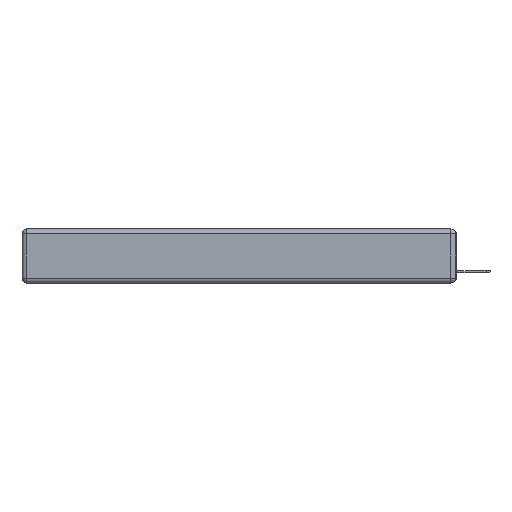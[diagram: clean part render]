
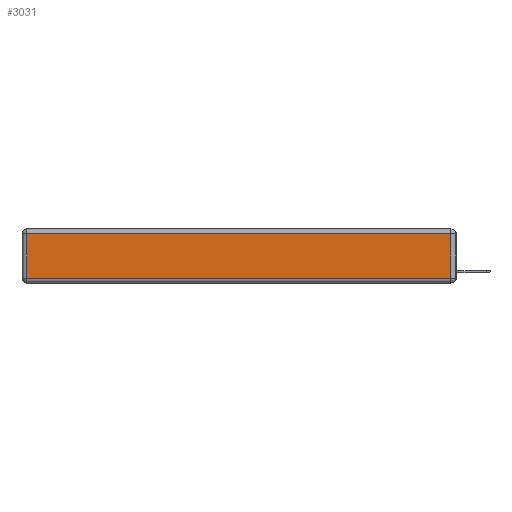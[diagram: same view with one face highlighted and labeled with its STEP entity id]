
A CAD part, left-side view. The second image highlights one B-rep face of the part: STEP entity #3031.
In plain terms, the highlighted planar face has unit normal (-1, 0, 0).
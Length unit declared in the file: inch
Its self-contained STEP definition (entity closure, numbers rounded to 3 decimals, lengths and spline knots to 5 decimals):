
#930 = CARTESIAN_POINT ( 'NONE',  ( 0., 2.72, -0.343 ) ) ;
#2395 = LINE ( 'NONE', #15706, #4545 ) ;
#2981 = ORIENTED_EDGE ( 'NONE', *, *, #5300, .T. ) ;
#3031 = ADVANCED_FACE ( 'NONE', ( #9175 ), #5121, .T. ) ;
#3174 = CARTESIAN_POINT ( 'NONE',  ( 0., 2.75, -0.03 ) ) ;
#3621 = DIRECTION ( 'NONE',  ( 0., 0., 1. ) ) ;
#4376 = VECTOR ( 'NONE', #15679, 39.37008 ) ;
#4486 = VERTEX_POINT ( 'NONE', #12995 ) ;
#4545 = VECTOR ( 'NONE', #3621, 39.37008 ) ;
#4649 = CARTESIAN_POINT ( 'NONE',  ( 0., 2.72, -0.03 ) ) ;
#5081 = VERTEX_POINT ( 'NONE', #4649 ) ;
#5121 = PLANE ( 'NONE',  #7846 ) ;
#5136 = VECTOR ( 'NONE', #11130, 39.37008 ) ;
#5223 = CARTESIAN_POINT ( 'NONE',  ( 0., 2.72, -0.313 ) ) ;
#5300 = EDGE_CURVE ( 'NONE', #5081, #17437, #6591, .T. ) ;
#5303 = DIRECTION ( 'NONE',  ( 0., 0., 1. ) ) ;
#5324 = CARTESIAN_POINT ( 'NONE',  ( 0., 0.03, -0.03 ) ) ;
#6591 = LINE ( 'NONE', #930, #4376 ) ;
#7787 = EDGE_CURVE ( 'NONE', #17437, #4486, #16787, .T. ) ;
#7846 = AXIS2_PLACEMENT_3D ( 'NONE', #17409, #15794, #5303 ) ;
#9175 = FACE_OUTER_BOUND ( 'NONE', #10873, .T. ) ;
#9381 = VECTOR ( 'NONE', #11759, 39.37008 ) ;
#10376 = ORIENTED_EDGE ( 'NONE', *, *, #11260, .T. ) ;
#10873 = EDGE_LOOP ( 'NONE', ( #12950, #10376, #12218, #2981 ) ) ;
#11130 = DIRECTION ( 'NONE',  ( 0., 1., 0. ) ) ;
#11260 = EDGE_CURVE ( 'NONE', #4486, #12232, #2395, .T. ) ;
#11759 = DIRECTION ( 'NONE',  ( 0., -1., 0. ) ) ;
#12218 = ORIENTED_EDGE ( 'NONE', *, *, #12414, .T. ) ;
#12232 = VERTEX_POINT ( 'NONE', #5324 ) ;
#12414 = EDGE_CURVE ( 'NONE', #12232, #5081, #12438, .T. ) ;
#12438 = LINE ( 'NONE', #3174, #5136 ) ;
#12950 = ORIENTED_EDGE ( 'NONE', *, *, #7787, .T. ) ;
#12995 = CARTESIAN_POINT ( 'NONE',  ( 0., 0.03, -0.313 ) ) ;
#15679 = DIRECTION ( 'NONE',  ( 0., 0., -1. ) ) ;
#15706 = CARTESIAN_POINT ( 'NONE',  ( 0., 0.03, -0.343 ) ) ;
#15794 = DIRECTION ( 'NONE',  ( -1., 0., 0. ) ) ;
#16787 = LINE ( 'NONE', #17064, #9381 ) ;
#17064 = CARTESIAN_POINT ( 'NONE',  ( 0., 0., -0.313 ) ) ;
#17409 = CARTESIAN_POINT ( 'NONE',  ( 0., 0., -0.343 ) ) ;
#17437 = VERTEX_POINT ( 'NONE', #5223 ) ;
